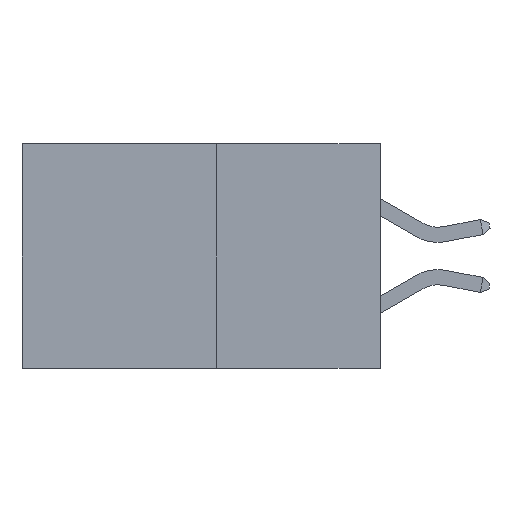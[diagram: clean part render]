
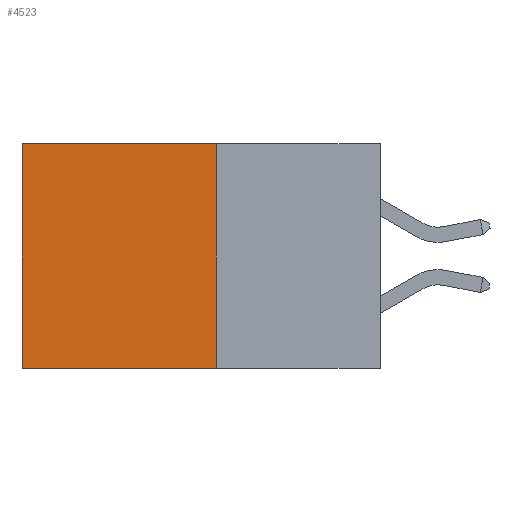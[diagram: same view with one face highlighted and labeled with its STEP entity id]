
A CAD part, left-side view. The second image highlights one B-rep face of the part: STEP entity #4523.
In plain terms, the highlighted planar face has unit normal (-1, 0, 0).
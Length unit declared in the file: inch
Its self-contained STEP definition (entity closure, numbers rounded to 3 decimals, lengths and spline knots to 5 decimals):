
#22 = DIRECTION ( 'NONE',  ( 0., 0., -1. ) ) ;
#468 = CARTESIAN_POINT ( 'NONE',  ( 0.277, 0.59, 0. ) ) ;
#720 = VECTOR ( 'NONE', #18894, 39.37008 ) ;
#4209 = EDGE_CURVE ( 'NONE', #7857, #18307, #16256, .T. ) ;
#4294 = EDGE_CURVE ( 'NONE', #26154, #7857, #17917, .T. ) ;
#4523 = ADVANCED_FACE ( 'NONE', ( #23260 ), #10633, .F. ) ;
#5885 = CARTESIAN_POINT ( 'NONE',  ( 0.277, 0.27, 0. ) ) ;
#6442 = CARTESIAN_POINT ( 'NONE',  ( 0.277, 0.59, -0.37 ) ) ;
#7857 = VERTEX_POINT ( 'NONE', #24970 ) ;
#8467 = ORIENTED_EDGE ( 'NONE', *, *, #4294, .F. ) ;
#9196 = VECTOR ( 'NONE', #23897, 39.37008 ) ;
#10420 = DIRECTION ( 'NONE',  ( 0., 0., -1. ) ) ;
#10473 = DIRECTION ( 'NONE',  ( 1., 0., 0. ) ) ;
#10483 = CARTESIAN_POINT ( 'NONE',  ( 0.277, 0.27, -0.37 ) ) ;
#10633 = PLANE ( 'NONE',  #17987 ) ;
#11736 = CARTESIAN_POINT ( 'NONE',  ( 0.277, 0.27, 0. ) ) ;
#13310 = ORIENTED_EDGE ( 'NONE', *, *, #26530, .T. ) ;
#13972 = EDGE_LOOP ( 'NONE', ( #21886, #20697, #8467, #13310 ) ) ;
#15404 = VERTEX_POINT ( 'NONE', #468 ) ;
#16256 = LINE ( 'NONE', #25176, #9196 ) ;
#17040 = VECTOR ( 'NONE', #22, 39.37008 ) ;
#17917 = LINE ( 'NONE', #19045, #720 ) ;
#17987 = AXIS2_PLACEMENT_3D ( 'NONE', #10483, #10473, #10420 ) ;
#18307 = VERTEX_POINT ( 'NONE', #21051 ) ;
#18894 = DIRECTION ( 'NONE',  ( 0., 0., -1. ) ) ;
#19045 = CARTESIAN_POINT ( 'NONE',  ( 0.277, 0.27, -0.37 ) ) ;
#20697 = ORIENTED_EDGE ( 'NONE', *, *, #4209, .F. ) ;
#20805 = VECTOR ( 'NONE', #23077, 39.37008 ) ;
#21051 = CARTESIAN_POINT ( 'NONE',  ( 0.277, 0.59, -0.37 ) ) ;
#21175 = EDGE_CURVE ( 'NONE', #15404, #18307, #24082, .T. ) ;
#21463 = LINE ( 'NONE', #5885, #20805 ) ;
#21886 = ORIENTED_EDGE ( 'NONE', *, *, #21175, .T. ) ;
#23077 = DIRECTION ( 'NONE',  ( 0., 1., 0. ) ) ;
#23260 = FACE_OUTER_BOUND ( 'NONE', #13972, .T. ) ;
#23897 = DIRECTION ( 'NONE',  ( 0., 1., 0. ) ) ;
#24082 = LINE ( 'NONE', #6442, #17040 ) ;
#24970 = CARTESIAN_POINT ( 'NONE',  ( 0.277, 0.27, -0.37 ) ) ;
#25176 = CARTESIAN_POINT ( 'NONE',  ( 0.277, 0.27, -0.37 ) ) ;
#26154 = VERTEX_POINT ( 'NONE', #11736 ) ;
#26530 = EDGE_CURVE ( 'NONE', #26154, #15404, #21463, .T. ) ;
